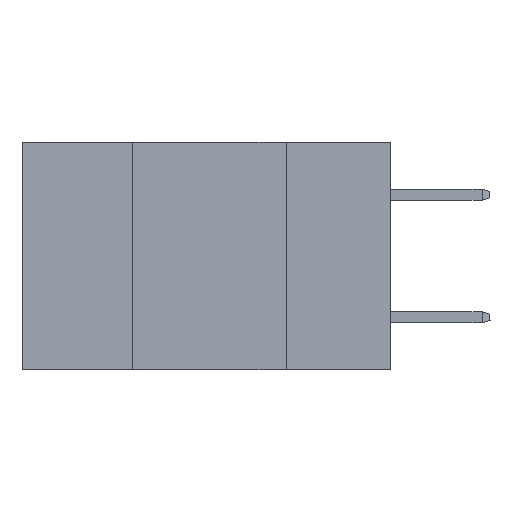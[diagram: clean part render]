
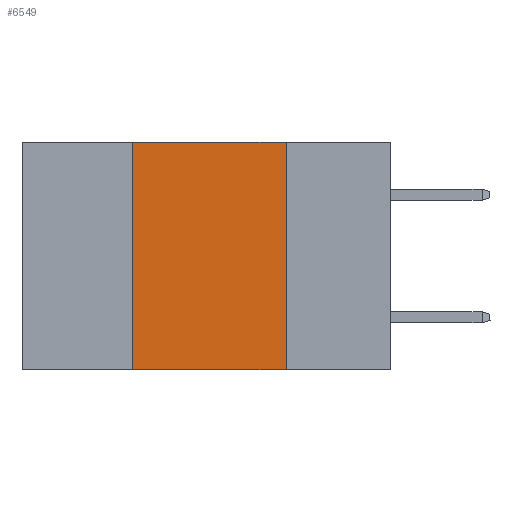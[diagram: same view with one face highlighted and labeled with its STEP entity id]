
A CAD part, left-side view. The second image highlights one B-rep face of the part: STEP entity #6549.
In plain terms, the highlighted planar face has unit normal (-1, 0, 0).
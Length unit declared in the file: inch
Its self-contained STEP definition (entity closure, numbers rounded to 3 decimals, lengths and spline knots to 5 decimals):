
#1440 = CARTESIAN_POINT ( 'NONE',  ( 0., 0.42, -0.37 ) ) ;
#2168 = VECTOR ( 'NONE', #13736, 39.37008 ) ;
#2457 = CARTESIAN_POINT ( 'NONE',  ( 0., 0.42, 0. ) ) ;
#3417 = LINE ( 'NONE', #23892, #2168 ) ;
#3447 = LINE ( 'NONE', #7093, #13468 ) ;
#4243 = DIRECTION ( 'NONE',  ( 0., -1., 0. ) ) ;
#4544 = VERTEX_POINT ( 'NONE', #7843 ) ;
#4973 = EDGE_CURVE ( 'NONE', #24832, #4544, #21486, .T. ) ;
#6148 = CARTESIAN_POINT ( 'NONE',  ( 0., 0.6, 0. ) ) ;
#6549 = ADVANCED_FACE ( 'NONE', ( #12108 ), #12906, .F. ) ;
#7093 = CARTESIAN_POINT ( 'NONE',  ( 0., 0.6, -0.37 ) ) ;
#7578 = CARTESIAN_POINT ( 'NONE',  ( 0., 0.42, 0. ) ) ;
#7843 = CARTESIAN_POINT ( 'NONE',  ( 0., 0.17, 0. ) ) ;
#8696 = VERTEX_POINT ( 'NONE', #1440 ) ;
#8930 = DIRECTION ( 'NONE',  ( 0., -1., 0. ) ) ;
#12108 = FACE_OUTER_BOUND ( 'NONE', #22269, .T. ) ;
#12233 = VERTEX_POINT ( 'NONE', #13713 ) ;
#12906 = PLANE ( 'NONE',  #23257 ) ;
#13468 = VECTOR ( 'NONE', #8930, 39.37008 ) ;
#13713 = CARTESIAN_POINT ( 'NONE',  ( 0., 0.17, -0.37 ) ) ;
#13736 = DIRECTION ( 'NONE',  ( 0., 0., -1. ) ) ;
#16077 = ORIENTED_EDGE ( 'NONE', *, *, #20494, .F. ) ;
#17517 = EDGE_CURVE ( 'NONE', #8696, #12233, #3447, .T. ) ;
#17810 = DIRECTION ( 'NONE',  ( 1., 0., 0. ) ) ;
#19297 = CARTESIAN_POINT ( 'NONE',  ( 0., 0.6, 0. ) ) ;
#19321 = ORIENTED_EDGE ( 'NONE', *, *, #17517, .T. ) ;
#20228 = DIRECTION ( 'NONE',  ( 0., 0., 1. ) ) ;
#20426 = ORIENTED_EDGE ( 'NONE', *, *, #21792, .F. ) ;
#20494 = EDGE_CURVE ( 'NONE', #8696, #24832, #20650, .T. ) ;
#20650 = LINE ( 'NONE', #2457, #23201 ) ;
#21486 = LINE ( 'NONE', #6148, #24031 ) ;
#21792 = EDGE_CURVE ( 'NONE', #4544, #12233, #3417, .T. ) ;
#22269 = EDGE_LOOP ( 'NONE', ( #20426, #25361, #16077, #19321 ) ) ;
#23201 = VECTOR ( 'NONE', #20228, 39.37008 ) ;
#23257 = AXIS2_PLACEMENT_3D ( 'NONE', #19297, #17810, #23453 ) ;
#23453 = DIRECTION ( 'NONE',  ( 0., 0., -1. ) ) ;
#23892 = CARTESIAN_POINT ( 'NONE',  ( 0., 0.17, 0. ) ) ;
#24031 = VECTOR ( 'NONE', #4243, 39.37008 ) ;
#24832 = VERTEX_POINT ( 'NONE', #7578 ) ;
#25361 = ORIENTED_EDGE ( 'NONE', *, *, #4973, .F. ) ;
